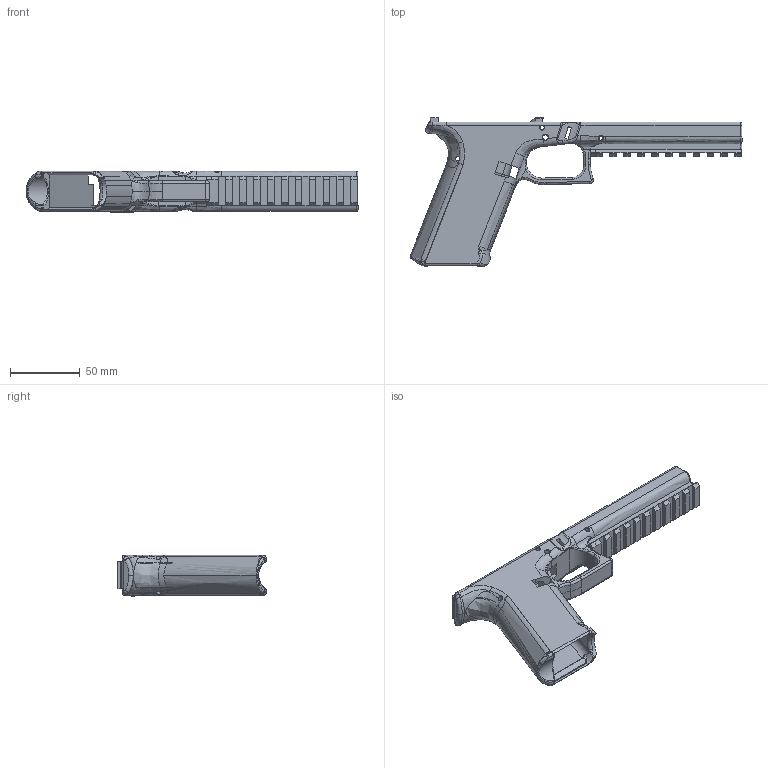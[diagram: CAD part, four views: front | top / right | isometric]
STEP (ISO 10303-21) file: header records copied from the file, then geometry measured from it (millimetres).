
FILE_DESCRIPTION(/* description */ (''),/* implementation_level */ '2;1');
FILE_NAME(/* name */ 'G17L PDW 3 Frame.step',/* time_stamp */ '2021-05-20T09:22:46-06:00',/* author */ (''),/* organization */ (''),/* preprocessor_version */ 'ST-DEVELOPER v18.1',/* originating_system */ 'Autodesk Translation Framework v10.6.0.1341',/* authorisation */ '');
FILE_SCHEMA (('AUTOMOTIVE_DESIGN { 1 0 10303 214 3 1 1 }'));
Products named in the file (1): G17L PDW 3
Bounding box: 238.63 x 106.5 x 29.84 mm (x, y, z)
Volume: 119302.8 mm3; surface area: 55400.4 mm2
Topology: 1 solids, 4 shells, 739 faces, 2061 edges, 1301 vertices
Faces by surface type: plane 306, bspline 260, cylinder 131, torus 21, sphere 14, cone 7
Full cylindrical faces by diameter (mm): 2 x1, 3 x4, 3.2 x2, 4 x2
Entity records: 49119 total; most frequent: CARTESIAN_POINT 31723, ORIENTED_EDGE 4104, DIRECTION 2979, EDGE_CURVE 2052, VERTEX_POINT 1302, LINE 1017, VECTOR 1017, AXIS2_PLACEMENT_3D 981
